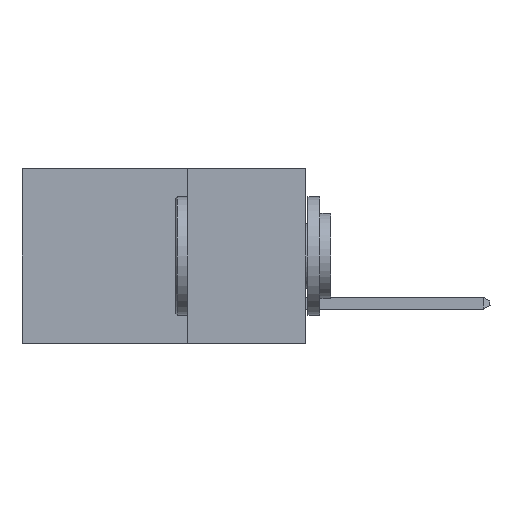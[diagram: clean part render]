
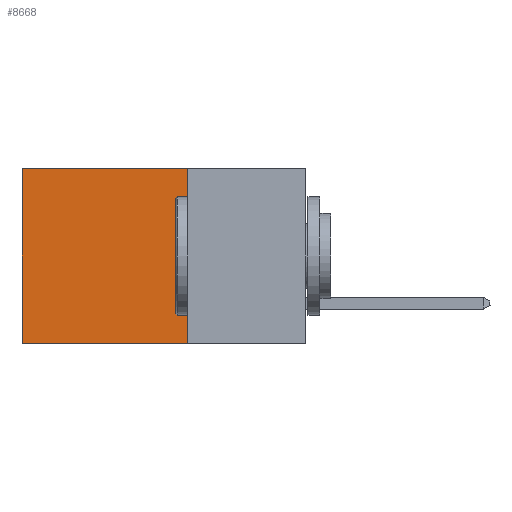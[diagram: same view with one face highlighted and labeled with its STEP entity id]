
A CAD part, left-side view. The second image highlights one B-rep face of the part: STEP entity #8668.
In plain terms, the highlighted planar face has unit normal (-1, 0, 0).
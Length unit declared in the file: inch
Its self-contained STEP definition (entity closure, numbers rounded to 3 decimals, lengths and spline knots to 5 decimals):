
#416 = CARTESIAN_POINT ( 'NONE',  ( 0.298, 0.25, 0. ) ) ;
#444 = AXIS2_PLACEMENT_3D ( 'NONE', #5966, #17517, #7630 ) ;
#705 = LINE ( 'NONE', #12054, #9259 ) ;
#1830 = CARTESIAN_POINT ( 'NONE',  ( 0.298, 0.6, 0. ) ) ;
#2325 = EDGE_LOOP ( 'NONE', ( #13303, #11443, #3363, #11073 ) ) ;
#2921 = FACE_OUTER_BOUND ( 'NONE', #2325, .T. ) ;
#3363 = ORIENTED_EDGE ( 'NONE', *, *, #11487, .F. ) ;
#3710 = VERTEX_POINT ( 'NONE', #9819 ) ;
#5966 = CARTESIAN_POINT ( 'NONE',  ( 0.298, 0.25, 0. ) ) ;
#7630 = DIRECTION ( 'NONE',  ( 0., 0., -1. ) ) ;
#8602 = DIRECTION ( 'NONE',  ( 0., 1., 0. ) ) ;
#8668 = ADVANCED_FACE ( 'NONE', ( #2921 ), #15878, .F. ) ;
#8761 = LINE ( 'NONE', #10853, #10278 ) ;
#9259 = VECTOR ( 'NONE', #8602, 39.37008 ) ;
#9680 = VECTOR ( 'NONE', #11845, 39.37008 ) ;
#9819 = CARTESIAN_POINT ( 'NONE',  ( 0.298, 0.25, 0. ) ) ;
#10278 = VECTOR ( 'NONE', #16067, 39.37008 ) ;
#10524 = CARTESIAN_POINT ( 'NONE',  ( 0.298, 0.6, -0.37 ) ) ;
#10853 = CARTESIAN_POINT ( 'NONE',  ( 0.298, 0.25, 0. ) ) ;
#10864 = EDGE_CURVE ( 'NONE', #3710, #17221, #8761, .T. ) ;
#11073 = ORIENTED_EDGE ( 'NONE', *, *, #10864, .T. ) ;
#11443 = ORIENTED_EDGE ( 'NONE', *, *, #11449, .F. ) ;
#11449 = EDGE_CURVE ( 'NONE', #15644, #20465, #705, .T. ) ;
#11487 = EDGE_CURVE ( 'NONE', #3710, #15644, #17498, .T. ) ;
#11845 = DIRECTION ( 'NONE',  ( 0., 0., -1. ) ) ;
#12054 = CARTESIAN_POINT ( 'NONE',  ( 0.298, 0.25, -0.37 ) ) ;
#13113 = VECTOR ( 'NONE', #18704, 39.37008 ) ;
#13303 = ORIENTED_EDGE ( 'NONE', *, *, #14720, .T. ) ;
#14720 = EDGE_CURVE ( 'NONE', #17221, #20465, #17677, .T. ) ;
#15644 = VERTEX_POINT ( 'NONE', #19158 ) ;
#15878 = PLANE ( 'NONE',  #444 ) ;
#16067 = DIRECTION ( 'NONE',  ( 0., 1., 0. ) ) ;
#17221 = VERTEX_POINT ( 'NONE', #1830 ) ;
#17498 = LINE ( 'NONE', #416, #13113 ) ;
#17517 = DIRECTION ( 'NONE',  ( 1., 0., 0. ) ) ;
#17677 = LINE ( 'NONE', #18436, #9680 ) ;
#18436 = CARTESIAN_POINT ( 'NONE',  ( 0.298, 0.6, 0. ) ) ;
#18704 = DIRECTION ( 'NONE',  ( 0., 0., -1. ) ) ;
#19158 = CARTESIAN_POINT ( 'NONE',  ( 0.298, 0.25, -0.37 ) ) ;
#20465 = VERTEX_POINT ( 'NONE', #10524 ) ;
